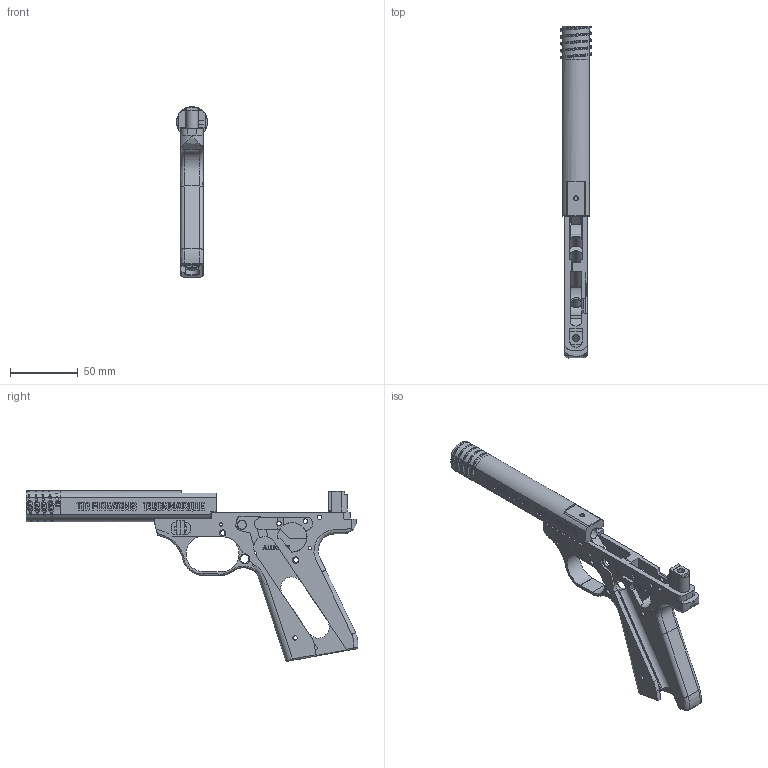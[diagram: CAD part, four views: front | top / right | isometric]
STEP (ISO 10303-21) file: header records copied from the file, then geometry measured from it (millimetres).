
FILE_DESCRIPTION(/* description */ (''),/* implementation_level */ '2;1');
FILE_NAME(/* name */ 'DBuckmarque V1.0.step',/* time_stamp */ '2022-04-28T13:21:46-07:00',/* author */ (''),/* organization */ (''),/* preprocessor_version */ 'ST-DEVELOPER v18.1',/* originating_system */ 'Autodesk Translation Framework v10.14.0.1471',/* authorisation */ '');
FILE_SCHEMA (('AUTOMOTIVE_DESIGN { 1 0 10303 214 3 1 1 }'));
Products named in the file (3): Browning Buckmark v3; Core Frame; Add On Printable Pieces
Assembly tree (2 placements, depth 2):
  Browning Buckmark v3
    Core Frame
    Add On Printable Pieces
Bounding box: 23.04 x 244.04 x 125.56 mm (x, y, z)
Volume: 152847.2 mm3; surface area: 66777.4 mm2
Topology: 5 solids, 6 shells, 1340 faces, 3643 edges, 2397 vertices
Faces by surface type: plane 1141, cylinder 134, bspline 48, torus 10, cone 7
Full cylindrical faces by diameter (mm): 1.4 x1, 2.5 x3, 3.15 x2, 3.2 x1, 3.35 x6, 3.5 x2, 3.6 x5, 4.6 x1, 5 x1, 5.9 x1, 6 x1, 6.4 x1, 6.45 x1, 6.5 x3, 6.6 x1, 7.68 x1, 8 x1, 8.2 x1, 8.5 x1, 9.5 x1, 23.048 x4
Entity records: 54170 total; most frequent: CARTESIAN_POINT 20366, ORIENTED_EDGE 7252, DIRECTION 6397, EDGE_CURVE 3626, LINE 3109, VECTOR 3109, VERTEX_POINT 2397, AXIS2_PLACEMENT_3D 1644
